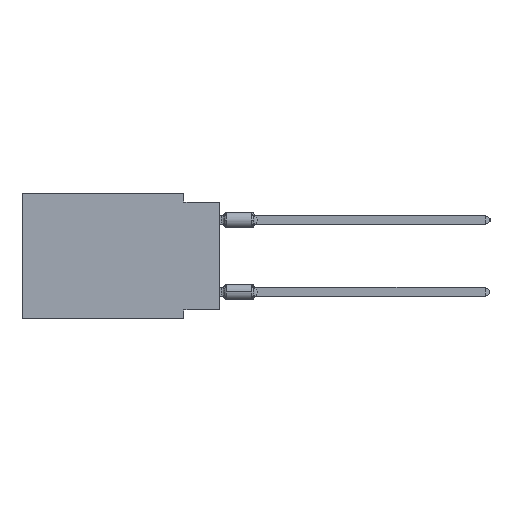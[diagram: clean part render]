
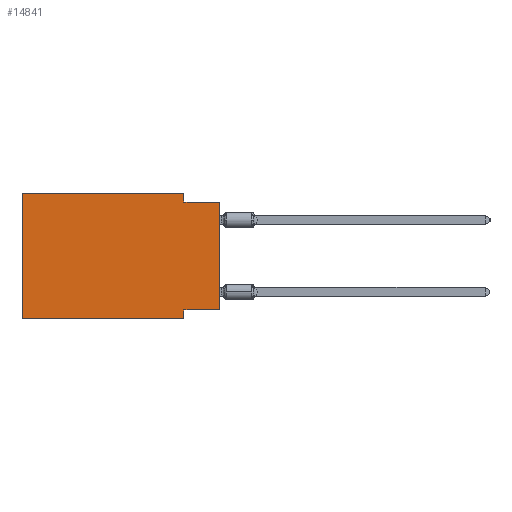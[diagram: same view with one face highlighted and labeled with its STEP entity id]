
A CAD part, left-side view. The second image highlights one B-rep face of the part: STEP entity #14841.
In plain terms, the highlighted planar face has unit normal (-1, 0, 0).
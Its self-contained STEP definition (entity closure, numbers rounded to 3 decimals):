
#94 = CARTESIAN_POINT ( 'NONE',  ( 0., 0., -8.255 ) ) ;
#1863 = DIRECTION ( 'NONE',  ( 0., 0., 1. ) ) ;
#2121 = ORIENTED_EDGE ( 'NONE', *, *, #19502, .F. ) ;
#2836 = CARTESIAN_POINT ( 'NONE',  ( 0., 13.97, 0. ) ) ;
#3330 = LINE ( 'NONE', #58449, #60830 ) ;
#5001 = CARTESIAN_POINT ( 'NONE',  ( 0., 0., -0.635 ) ) ;
#5111 = CARTESIAN_POINT ( 'NONE',  ( 0., 13.97, 0. ) ) ;
#6770 = CARTESIAN_POINT ( 'NONE',  ( 0., 2.54, -0.635 ) ) ;
#7567 = CARTESIAN_POINT ( 'NONE',  ( 0., 2.54, -8.89 ) ) ;
#8220 = DIRECTION ( 'NONE',  ( 0., -1., 0. ) ) ;
#8698 = EDGE_CURVE ( 'NONE', #17247, #34369, #50998, .T. ) ;
#9855 = DIRECTION ( 'NONE',  ( 0., 0., -1. ) ) ;
#10997 = DIRECTION ( 'NONE',  ( 0., 0., 1. ) ) ;
#11324 = ORIENTED_EDGE ( 'NONE', *, *, #59905, .F. ) ;
#12544 = CARTESIAN_POINT ( 'NONE',  ( 0., 13.97, -8.89 ) ) ;
#13337 = VERTEX_POINT ( 'NONE', #6770 ) ;
#13501 = LINE ( 'NONE', #42878, #29218 ) ;
#14841 = ADVANCED_FACE ( 'NONE', ( #25518 ), #59433, .F. ) ;
#15210 = VECTOR ( 'NONE', #1863, 1000. ) ;
#16519 = ORIENTED_EDGE ( 'NONE', *, *, #44635, .T. ) ;
#17247 = VERTEX_POINT ( 'NONE', #94 ) ;
#17367 = VECTOR ( 'NONE', #20668, 1000. ) ;
#19502 = EDGE_CURVE ( 'NONE', #20008, #55113, #19822, .T. ) ;
#19822 = LINE ( 'NONE', #2836, #15210 ) ;
#20008 = VERTEX_POINT ( 'NONE', #12544 ) ;
#20668 = DIRECTION ( 'NONE',  ( 0., 1., 0. ) ) ;
#21325 = EDGE_CURVE ( 'NONE', #20008, #33835, #13501, .T. ) ;
#22272 = CARTESIAN_POINT ( 'NONE',  ( 0., 2.54, 0. ) ) ;
#23025 = ORIENTED_EDGE ( 'NONE', *, *, #21325, .T. ) ;
#23210 = VECTOR ( 'NONE', #8220, 1000. ) ;
#23238 = DIRECTION ( 'NONE',  ( 0., -1., 0. ) ) ;
#25518 = FACE_OUTER_BOUND ( 'NONE', #46140, .T. ) ;
#27467 = ORIENTED_EDGE ( 'NONE', *, *, #63152, .F. ) ;
#27502 = EDGE_CURVE ( 'NONE', #34369, #33835, #52248, .T. ) ;
#27801 = VECTOR ( 'NONE', #10997, 1000. ) ;
#29218 = VECTOR ( 'NONE', #63725, 1000. ) ;
#30458 = CARTESIAN_POINT ( 'NONE',  ( 0., 0., -8.255 ) ) ;
#31076 = ORIENTED_EDGE ( 'NONE', *, *, #27502, .F. ) ;
#32023 = CARTESIAN_POINT ( 'NONE',  ( 0., 2.54, 0. ) ) ;
#33835 = VERTEX_POINT ( 'NONE', #48042 ) ;
#34369 = VERTEX_POINT ( 'NONE', #64204 ) ;
#39743 = VECTOR ( 'NONE', #57768, 1000. ) ;
#42878 = CARTESIAN_POINT ( 'NONE',  ( 0., 13.97, -8.89 ) ) ;
#44635 = EDGE_CURVE ( 'NONE', #17247, #50049, #55364, .T. ) ;
#45197 = EDGE_CURVE ( 'NONE', #59775, #13337, #47670, .T. ) ;
#46140 = EDGE_LOOP ( 'NONE', ( #16519, #27467, #60163, #11324, #2121, #23025, #31076, #62425 ) ) ;
#47670 = LINE ( 'NONE', #32023, #39743 ) ;
#48042 = CARTESIAN_POINT ( 'NONE',  ( 0., 2.54, -8.89 ) ) ;
#49982 = CARTESIAN_POINT ( 'NONE',  ( 0., 13.97, 0. ) ) ;
#50049 = VERTEX_POINT ( 'NONE', #5001 ) ;
#50998 = LINE ( 'NONE', #30458, #17367 ) ;
#52248 = LINE ( 'NONE', #7567, #55326 ) ;
#52906 = LINE ( 'NONE', #58123, #23210 ) ;
#53129 = AXIS2_PLACEMENT_3D ( 'NONE', #49982, #64012, #9855 ) ;
#55113 = VERTEX_POINT ( 'NONE', #5111 ) ;
#55326 = VECTOR ( 'NONE', #62054, 1000. ) ;
#55364 = LINE ( 'NONE', #60574, #27801 ) ;
#57768 = DIRECTION ( 'NONE',  ( 0., 0., -1. ) ) ;
#58123 = CARTESIAN_POINT ( 'NONE',  ( 0., 13.97, 0. ) ) ;
#58449 = CARTESIAN_POINT ( 'NONE',  ( 0., 0., -0.635 ) ) ;
#59433 = PLANE ( 'NONE',  #53129 ) ;
#59775 = VERTEX_POINT ( 'NONE', #22272 ) ;
#59905 = EDGE_CURVE ( 'NONE', #55113, #59775, #52906, .T. ) ;
#60163 = ORIENTED_EDGE ( 'NONE', *, *, #45197, .F. ) ;
#60574 = CARTESIAN_POINT ( 'NONE',  ( 0., 0., 0. ) ) ;
#60830 = VECTOR ( 'NONE', #23238, 1000. ) ;
#62054 = DIRECTION ( 'NONE',  ( 0., 0., -1. ) ) ;
#62425 = ORIENTED_EDGE ( 'NONE', *, *, #8698, .F. ) ;
#63152 = EDGE_CURVE ( 'NONE', #13337, #50049, #3330, .T. ) ;
#63725 = DIRECTION ( 'NONE',  ( 0., -1., 0. ) ) ;
#64012 = DIRECTION ( 'NONE',  ( 1., 0., 0. ) ) ;
#64204 = CARTESIAN_POINT ( 'NONE',  ( 0., 2.54, -8.255 ) ) ;
